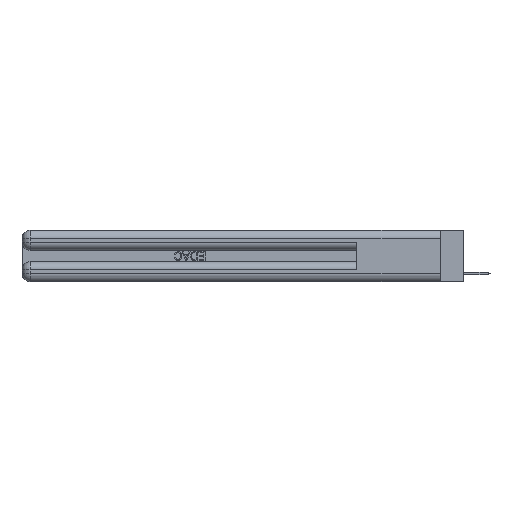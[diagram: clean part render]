
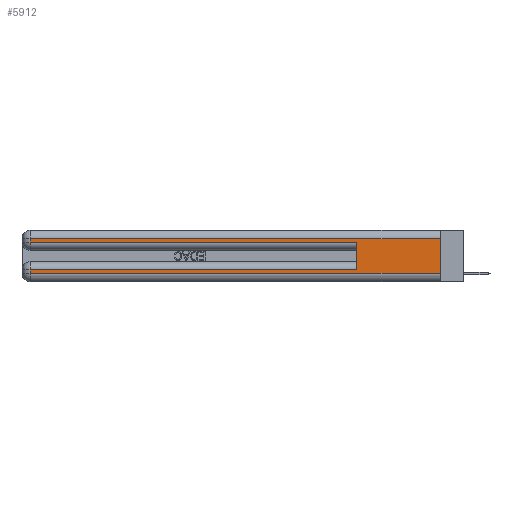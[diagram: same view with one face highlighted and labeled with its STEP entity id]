
A CAD part, left-side view. The second image highlights one B-rep face of the part: STEP entity #5912.
In plain terms, the highlighted planar face has unit normal (-1, 0, 0).
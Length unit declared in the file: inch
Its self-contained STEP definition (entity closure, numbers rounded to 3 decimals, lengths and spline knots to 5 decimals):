
#179 = EDGE_CURVE ( 'NONE', #6696, #30802, #1182, .T. ) ;
#450 = ORIENTED_EDGE ( 'NONE', *, *, #25923, .T. ) ;
#518 = VERTEX_POINT ( 'NONE', #9857 ) ;
#887 = EDGE_CURVE ( 'NONE', #518, #13885, #7205, .T. ) ;
#1182 = LINE ( 'NONE', #18730, #20074 ) ;
#1625 = AXIS2_PLACEMENT_3D ( 'NONE', #3399, #17698, #8347 ) ;
#2000 = DIRECTION ( 'NONE',  ( 0., 0., 1. ) ) ;
#2428 = CARTESIAN_POINT ( 'NONE',  ( 0., 0., 0.31 ) ) ;
#3399 = CARTESIAN_POINT ( 'NONE',  ( 0., 0., 0.37 ) ) ;
#3766 = EDGE_LOOP ( 'NONE', ( #30106, #9673, #20651, #5256, #16540, #7820, #450, #23395 ) ) ;
#3901 = DIRECTION ( 'NONE',  ( 0., -1., 0. ) ) ;
#5256 = ORIENTED_EDGE ( 'NONE', *, *, #8323, .T. ) ;
#5706 = CARTESIAN_POINT ( 'NONE',  ( 0., 2.94, 0.085 ) ) ;
#5743 = VECTOR ( 'NONE', #7859, 39.37008 ) ;
#5912 = ADVANCED_FACE ( 'NONE', ( #30782 ), #10477, .F. ) ;
#6696 = VERTEX_POINT ( 'NONE', #16089 ) ;
#6783 = LINE ( 'NONE', #25118, #16705 ) ;
#7205 = LINE ( 'NONE', #2428, #12796 ) ;
#7820 = ORIENTED_EDGE ( 'NONE', *, *, #18066, .T. ) ;
#7859 = DIRECTION ( 'NONE',  ( 0., 0., -1. ) ) ;
#7980 = VECTOR ( 'NONE', #22241, 39.37008 ) ;
#8323 = EDGE_CURVE ( 'NONE', #20066, #20831, #29000, .T. ) ;
#8347 = DIRECTION ( 'NONE',  ( 0., 0., -1. ) ) ;
#8398 = EDGE_CURVE ( 'NONE', #13885, #20066, #16891, .T. ) ;
#9054 = CARTESIAN_POINT ( 'NONE',  ( 0., 0.6, 0.285 ) ) ;
#9673 = ORIENTED_EDGE ( 'NONE', *, *, #887, .T. ) ;
#9857 = CARTESIAN_POINT ( 'NONE',  ( 0., 0., 0.31 ) ) ;
#10450 = VECTOR ( 'NONE', #27230, 39.37008 ) ;
#10477 = PLANE ( 'NONE',  #1625 ) ;
#11354 = VECTOR ( 'NONE', #3901, 39.37008 ) ;
#11876 = VECTOR ( 'NONE', #18676, 39.37008 ) ;
#12796 = VECTOR ( 'NONE', #24744, 39.37008 ) ;
#13115 = CARTESIAN_POINT ( 'NONE',  ( 0., 0., 0.06 ) ) ;
#13885 = VERTEX_POINT ( 'NONE', #30003 ) ;
#16089 = CARTESIAN_POINT ( 'NONE',  ( 0., 2.94, 0.06 ) ) ;
#16540 = ORIENTED_EDGE ( 'NONE', *, *, #22992, .F. ) ;
#16705 = VECTOR ( 'NONE', #2000, 39.37008 ) ;
#16891 = LINE ( 'NONE', #31631, #11876 ) ;
#17698 = DIRECTION ( 'NONE',  ( 1., 0., 0. ) ) ;
#18066 = EDGE_CURVE ( 'NONE', #20884, #23721, #32165, .T. ) ;
#18676 = DIRECTION ( 'NONE',  ( 0., 0., -1. ) ) ;
#18730 = CARTESIAN_POINT ( 'NONE',  ( 0., 0., 0.06 ) ) ;
#20066 = VERTEX_POINT ( 'NONE', #28642 ) ;
#20074 = VECTOR ( 'NONE', #23813, 39.37008 ) ;
#20301 = LINE ( 'NONE', #30277, #5743 ) ;
#20651 = ORIENTED_EDGE ( 'NONE', *, *, #8398, .T. ) ;
#20831 = VERTEX_POINT ( 'NONE', #9054 ) ;
#20884 = VERTEX_POINT ( 'NONE', #28545 ) ;
#21788 = CARTESIAN_POINT ( 'NONE',  ( 0., 0., 0.285 ) ) ;
#22241 = DIRECTION ( 'NONE',  ( 0., 0., -1. ) ) ;
#22992 = EDGE_CURVE ( 'NONE', #20884, #20831, #6783, .T. ) ;
#23395 = ORIENTED_EDGE ( 'NONE', *, *, #179, .T. ) ;
#23721 = VERTEX_POINT ( 'NONE', #5706 ) ;
#23813 = DIRECTION ( 'NONE',  ( 0., -1., 0. ) ) ;
#24744 = DIRECTION ( 'NONE',  ( 0., 1., 0. ) ) ;
#25003 = CARTESIAN_POINT ( 'NONE',  ( 0., 0., 0.37 ) ) ;
#25118 = CARTESIAN_POINT ( 'NONE',  ( 0., 0.6, 0.145 ) ) ;
#25923 = EDGE_CURVE ( 'NONE', #23721, #6696, #20301, .T. ) ;
#26033 = LINE ( 'NONE', #25003, #7980 ) ;
#27230 = DIRECTION ( 'NONE',  ( 0., 1., 0. ) ) ;
#28545 = CARTESIAN_POINT ( 'NONE',  ( 0., 0.6, 0.085 ) ) ;
#28642 = CARTESIAN_POINT ( 'NONE',  ( 0., 2.94, 0.285 ) ) ;
#29000 = LINE ( 'NONE', #21788, #11354 ) ;
#30003 = CARTESIAN_POINT ( 'NONE',  ( 0., 2.94, 0.31 ) ) ;
#30106 = ORIENTED_EDGE ( 'NONE', *, *, #31004, .F. ) ;
#30277 = CARTESIAN_POINT ( 'NONE',  ( 0., 2.94, 0.37 ) ) ;
#30782 = FACE_OUTER_BOUND ( 'NONE', #3766, .T. ) ;
#30802 = VERTEX_POINT ( 'NONE', #13115 ) ;
#31004 = EDGE_CURVE ( 'NONE', #518, #30802, #26033, .T. ) ;
#31631 = CARTESIAN_POINT ( 'NONE',  ( 0., 2.94, 0.37 ) ) ;
#32165 = LINE ( 'NONE', #32317, #10450 ) ;
#32317 = CARTESIAN_POINT ( 'NONE',  ( 0., 0., 0.085 ) ) ;
